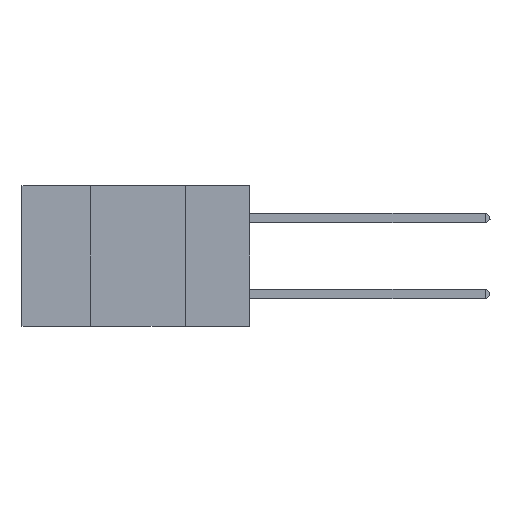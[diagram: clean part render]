
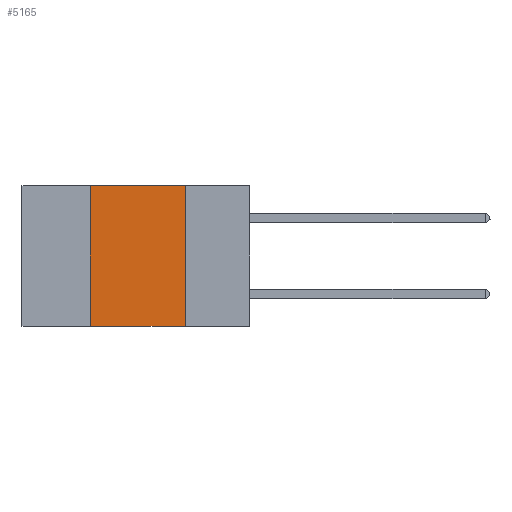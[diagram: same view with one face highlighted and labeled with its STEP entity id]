
A CAD part, left-side view. The second image highlights one B-rep face of the part: STEP entity #5165.
In plain terms, the highlighted planar face has unit normal (-1, 0, 0).
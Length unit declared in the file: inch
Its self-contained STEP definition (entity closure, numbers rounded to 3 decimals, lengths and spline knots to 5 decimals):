
#970 = DIRECTION ( 'NONE',  ( 1., 0., 0. ) ) ;
#1052 = VERTEX_POINT ( 'NONE', #3825 ) ;
#1060 = DIRECTION ( 'NONE',  ( 0., -1., 0. ) ) ;
#1338 = LINE ( 'NONE', #3021, #9567 ) ;
#1622 = VERTEX_POINT ( 'NONE', #6314 ) ;
#2209 = DIRECTION ( 'NONE',  ( 0., 0., -1. ) ) ;
#2255 = EDGE_LOOP ( 'NONE', ( #9628, #2440, #3982, #7480 ) ) ;
#2390 = AXIS2_PLACEMENT_3D ( 'NONE', #8467, #970, #4300 ) ;
#2440 = ORIENTED_EDGE ( 'NONE', *, *, #2688, .F. ) ;
#2587 = VERTEX_POINT ( 'NONE', #9874 ) ;
#2688 = EDGE_CURVE ( 'NONE', #2587, #1052, #4205, .T. ) ;
#3021 = CARTESIAN_POINT ( 'NONE',  ( 0., 0.17, 0. ) ) ;
#3310 = VECTOR ( 'NONE', #1060, 39.37008 ) ;
#3481 = DIRECTION ( 'NONE',  ( 0., -1., 0. ) ) ;
#3825 = CARTESIAN_POINT ( 'NONE',  ( 0., 0.17, 0. ) ) ;
#3943 = LINE ( 'NONE', #6457, #9396 ) ;
#3982 = ORIENTED_EDGE ( 'NONE', *, *, #7417, .F. ) ;
#4074 = VERTEX_POINT ( 'NONE', #8332 ) ;
#4205 = LINE ( 'NONE', #6674, #4930 ) ;
#4300 = DIRECTION ( 'NONE',  ( 0., 0., -1. ) ) ;
#4930 = VECTOR ( 'NONE', #3481, 39.37008 ) ;
#5165 = ADVANCED_FACE ( 'NONE', ( #7757 ), #5168, .F. ) ;
#5168 = PLANE ( 'NONE',  #2390 ) ;
#6091 = CARTESIAN_POINT ( 'NONE',  ( 0., 0.6, -0.37 ) ) ;
#6314 = CARTESIAN_POINT ( 'NONE',  ( 0., 0.17, -0.37 ) ) ;
#6457 = CARTESIAN_POINT ( 'NONE',  ( 0., 0.42, 0. ) ) ;
#6563 = EDGE_CURVE ( 'NONE', #1052, #1622, #1338, .T. ) ;
#6674 = CARTESIAN_POINT ( 'NONE',  ( 0., 0.6, 0. ) ) ;
#7417 = EDGE_CURVE ( 'NONE', #4074, #2587, #3943, .T. ) ;
#7480 = ORIENTED_EDGE ( 'NONE', *, *, #8139, .T. ) ;
#7757 = FACE_OUTER_BOUND ( 'NONE', #2255, .T. ) ;
#8139 = EDGE_CURVE ( 'NONE', #4074, #1622, #8560, .T. ) ;
#8332 = CARTESIAN_POINT ( 'NONE',  ( 0., 0.42, -0.37 ) ) ;
#8467 = CARTESIAN_POINT ( 'NONE',  ( 0., 0.6, 0. ) ) ;
#8560 = LINE ( 'NONE', #6091, #3310 ) ;
#9396 = VECTOR ( 'NONE', #10646, 39.37008 ) ;
#9567 = VECTOR ( 'NONE', #2209, 39.37008 ) ;
#9628 = ORIENTED_EDGE ( 'NONE', *, *, #6563, .F. ) ;
#9874 = CARTESIAN_POINT ( 'NONE',  ( 0., 0.42, 0. ) ) ;
#10646 = DIRECTION ( 'NONE',  ( 0., 0., 1. ) ) ;
